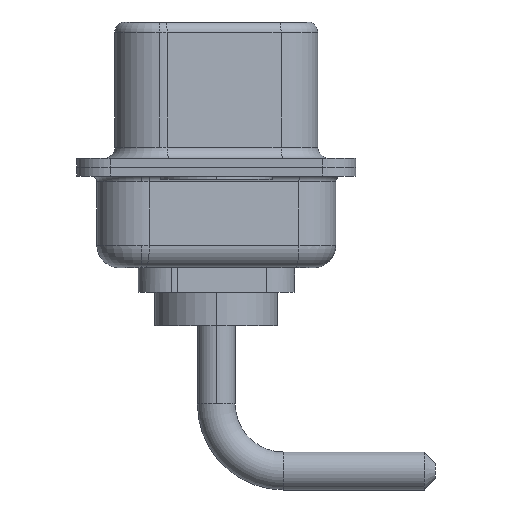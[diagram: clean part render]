
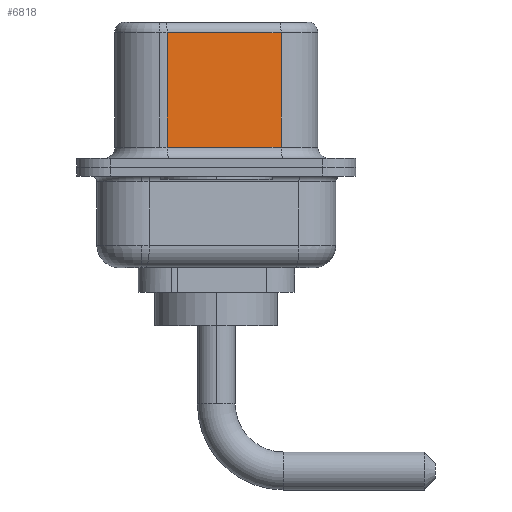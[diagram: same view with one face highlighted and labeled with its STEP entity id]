
A CAD part, left-side view. The second image highlights one B-rep face of the part: STEP entity #6818.
In plain terms, the highlighted planar face has unit normal (-0.985, -0.174, 0).
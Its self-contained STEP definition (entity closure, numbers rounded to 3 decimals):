
#370 = CARTESIAN_POINT ( 'NONE',  ( 3.655, 2.203, 0.9 ) ) ;
#506 = LINE ( 'NONE', #11187, #6205 ) ;
#1177 = LINE ( 'NONE', #9032, #6124 ) ;
#1470 = EDGE_CURVE ( 'NONE', #2783, #7483, #506, .T. ) ;
#1668 = CARTESIAN_POINT ( 'NONE',  ( 4.555, -2.897, 6.02 ) ) ;
#2783 = VERTEX_POINT ( 'NONE', #370 ) ;
#3118 = CARTESIAN_POINT ( 'NONE',  ( 4.555, -2.897, 6.52 ) ) ;
#3193 = ORIENTED_EDGE ( 'NONE', *, *, #3710, .T. ) ;
#3229 = DIRECTION ( 'NONE',  ( -0.174, 0.985, 0. ) ) ;
#3667 = DIRECTION ( 'NONE',  ( 0.174, -0.985, 0. ) ) ;
#3710 = EDGE_CURVE ( 'NONE', #6435, #10171, #8562, .T. ) ;
#4042 = ORIENTED_EDGE ( 'NONE', *, *, #10710, .F. ) ;
#4158 = CARTESIAN_POINT ( 'NONE',  ( 4.555, -2.897, 0.9 ) ) ;
#5605 = DIRECTION ( 'NONE',  ( 0., 0., -1. ) ) ;
#6003 = ORIENTED_EDGE ( 'NONE', *, *, #1470, .T. ) ;
#6124 = VECTOR ( 'NONE', #5605, 1000. ) ;
#6205 = VECTOR ( 'NONE', #3667, 1000. ) ;
#6435 = VERTEX_POINT ( 'NONE', #1668 ) ;
#6784 = FACE_OUTER_BOUND ( 'NONE', #7569, .T. ) ;
#6818 = ADVANCED_FACE ( 'NONE', ( #6784 ), #8956, .F. ) ;
#7051 = ORIENTED_EDGE ( 'NONE', *, *, #13093, .T. ) ;
#7057 = CARTESIAN_POINT ( 'NONE',  ( 4.555, -2.897, 6.52 ) ) ;
#7483 = VERTEX_POINT ( 'NONE', #4158 ) ;
#7569 = EDGE_LOOP ( 'NONE', ( #4042, #3193, #7051, #6003 ) ) ;
#7684 = CARTESIAN_POINT ( 'NONE',  ( 3.655, 2.203, 6.02 ) ) ;
#8492 = VECTOR ( 'NONE', #3229, 1000. ) ;
#8562 = LINE ( 'NONE', #12825, #8492 ) ;
#8956 = PLANE ( 'NONE',  #13228 ) ;
#9032 = CARTESIAN_POINT ( 'NONE',  ( 3.655, 2.203, 6.52 ) ) ;
#9554 = VECTOR ( 'NONE', #11750, 1000. ) ;
#10171 = VERTEX_POINT ( 'NONE', #7684 ) ;
#10710 = EDGE_CURVE ( 'NONE', #6435, #7483, #10910, .T. ) ;
#10910 = LINE ( 'NONE', #3118, #9554 ) ;
#11124 = DIRECTION ( 'NONE',  ( -0.174, 0.985, 0. ) ) ;
#11187 = CARTESIAN_POINT ( 'NONE',  ( 4.555, -2.897, 0.9 ) ) ;
#11750 = DIRECTION ( 'NONE',  ( 0., 0., -1. ) ) ;
#12825 = CARTESIAN_POINT ( 'NONE',  ( 4.555, -2.897, 6.02 ) ) ;
#13093 = EDGE_CURVE ( 'NONE', #10171, #2783, #1177, .T. ) ;
#13228 = AXIS2_PLACEMENT_3D ( 'NONE', #7057, #13431, #11124 ) ;
#13431 = DIRECTION ( 'NONE',  ( 0.985, 0.174, 0. ) ) ;
